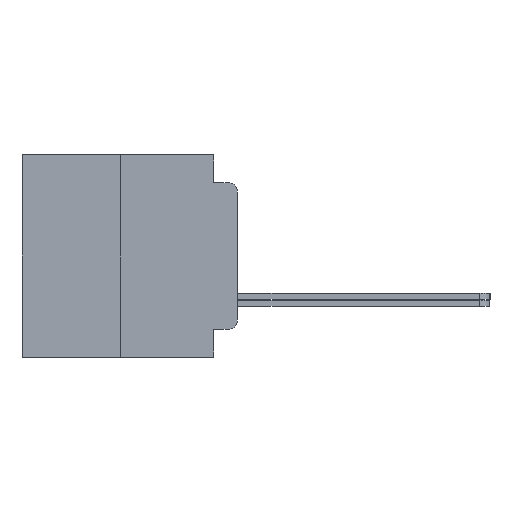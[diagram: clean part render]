
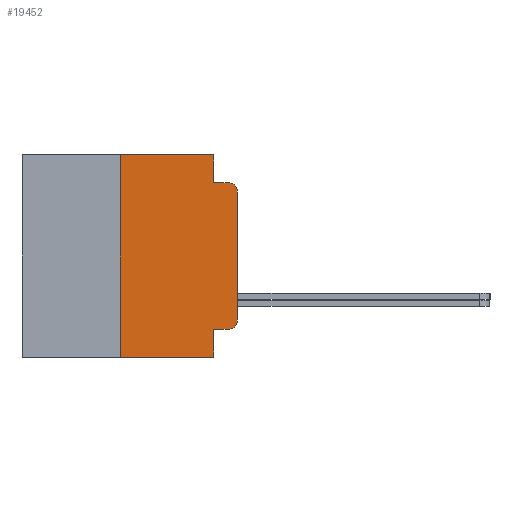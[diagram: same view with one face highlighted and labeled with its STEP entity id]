
A CAD part, left-side view. The second image highlights one B-rep face of the part: STEP entity #19452.
In plain terms, the highlighted planar face has unit normal (-1, 0, 0).
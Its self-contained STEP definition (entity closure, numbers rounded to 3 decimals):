
#220 = VECTOR ( 'NONE', #13989, 1000. ) ;
#304 = VERTEX_POINT ( 'NONE', #727 ) ;
#560 = CARTESIAN_POINT ( 'NONE',  ( -75.603, 0.508, 3.467 ) ) ;
#727 = CARTESIAN_POINT ( 'NONE',  ( -75.603, 1.295, 5.486 ) ) ;
#997 = VERTEX_POINT ( 'NONE', #19934 ) ;
#1401 = CARTESIAN_POINT ( 'NONE',  ( -75.603, 6.35, 5.486 ) ) ;
#2015 = LINE ( 'NONE', #21872, #22476 ) ;
#2050 = LINE ( 'NONE', #23682, #16627 ) ;
#2599 = LINE ( 'NONE', #22266, #8858 ) ;
#2803 = DIRECTION ( 'NONE',  ( 0., 0., -1. ) ) ;
#3021 = LINE ( 'NONE', #4930, #20056 ) ;
#3173 = DIRECTION ( 'NONE',  ( 0., 0., -1. ) ) ;
#4796 = CARTESIAN_POINT ( 'NONE',  ( -75.603, 6.35, -5.486 ) ) ;
#4930 = CARTESIAN_POINT ( 'NONE',  ( -75.603, 0., 5.486 ) ) ;
#5024 = LINE ( 'NONE', #7164, #17158 ) ;
#5097 = VECTOR ( 'NONE', #25494, 1000. ) ;
#5212 = PLANE ( 'NONE',  #24274 ) ;
#5493 = CARTESIAN_POINT ( 'NONE',  ( -75.603, 1.295, -3.975 ) ) ;
#5762 = CARTESIAN_POINT ( 'NONE',  ( -75.603, 1.295, -3.975 ) ) ;
#5811 = EDGE_CURVE ( 'NONE', #6834, #17138, #17463, .T. ) ;
#5921 = CARTESIAN_POINT ( 'NONE',  ( -75.603, 11.684, -5.486 ) ) ;
#6027 = CIRCLE ( 'NONE', #8150, 0.508 ) ;
#6270 = DIRECTION ( 'NONE',  ( 0., 0., -1. ) ) ;
#6372 = DIRECTION ( 'NONE',  ( 0., 0., -1. ) ) ;
#6834 = VERTEX_POINT ( 'NONE', #24407 ) ;
#7164 = CARTESIAN_POINT ( 'NONE',  ( -75.603, 1.295, 3.975 ) ) ;
#7718 = VERTEX_POINT ( 'NONE', #7725 ) ;
#7725 = CARTESIAN_POINT ( 'NONE',  ( -75.603, 0.508, -3.975 ) ) ;
#8150 = AXIS2_PLACEMENT_3D ( 'NONE', #14321, #11889, #3173 ) ;
#8215 = LINE ( 'NONE', #5921, #25603 ) ;
#8858 = VECTOR ( 'NONE', #6372, 1000. ) ;
#9662 = CARTESIAN_POINT ( 'NONE',  ( -75.603, 11.684, 5.486 ) ) ;
#10003 = DIRECTION ( 'NONE',  ( 0., -1., 0. ) ) ;
#10238 = EDGE_CURVE ( 'NONE', #304, #997, #2599, .T. ) ;
#11692 = ORIENTED_EDGE ( 'NONE', *, *, #5811, .T. ) ;
#11889 = DIRECTION ( 'NONE',  ( -1., 0., 0. ) ) ;
#11892 = DIRECTION ( 'NONE',  ( 0., 0., -1. ) ) ;
#12378 = CARTESIAN_POINT ( 'NONE',  ( -75.603, 1.295, -5.486 ) ) ;
#12383 = LINE ( 'NONE', #5493, #5097 ) ;
#12546 = ORIENTED_EDGE ( 'NONE', *, *, #21120, .T. ) ;
#13679 = EDGE_CURVE ( 'NONE', #23875, #15621, #8215, .T. ) ;
#13989 = DIRECTION ( 'NONE',  ( 0., 0., 1. ) ) ;
#14321 = CARTESIAN_POINT ( 'NONE',  ( -75.603, 0.508, -3.467 ) ) ;
#14332 = VERTEX_POINT ( 'NONE', #5762 ) ;
#14363 = VERTEX_POINT ( 'NONE', #1401 ) ;
#14420 = DIRECTION ( 'NONE',  ( 0., -1., 0. ) ) ;
#14686 = EDGE_CURVE ( 'NONE', #997, #17138, #5024, .T. ) ;
#15621 = VERTEX_POINT ( 'NONE', #12378 ) ;
#15919 = ORIENTED_EDGE ( 'NONE', *, *, #14686, .F. ) ;
#16088 = DIRECTION ( 'NONE',  ( -1., 0., 0. ) ) ;
#16627 = VECTOR ( 'NONE', #18845, 1000. ) ;
#17138 = VERTEX_POINT ( 'NONE', #26164 ) ;
#17158 = VECTOR ( 'NONE', #14420, 1000. ) ;
#17463 = CIRCLE ( 'NONE', #21462, 0.508 ) ;
#17610 = EDGE_CURVE ( 'NONE', #14363, #304, #2050, .T. ) ;
#18006 = ORIENTED_EDGE ( 'NONE', *, *, #21700, .F. ) ;
#18749 = VERTEX_POINT ( 'NONE', #21094 ) ;
#18845 = DIRECTION ( 'NONE',  ( 0., -1., 0. ) ) ;
#18940 = EDGE_CURVE ( 'NONE', #14332, #15621, #2015, .T. ) ;
#19056 = ORIENTED_EDGE ( 'NONE', *, *, #10238, .F. ) ;
#19164 = ORIENTED_EDGE ( 'NONE', *, *, #21260, .T. ) ;
#19452 = ADVANCED_FACE ( 'NONE', ( #22907 ), #5212, .F. ) ;
#19681 = ORIENTED_EDGE ( 'NONE', *, *, #23400, .T. ) ;
#19934 = CARTESIAN_POINT ( 'NONE',  ( -75.603, 1.295, 3.975 ) ) ;
#20056 = VECTOR ( 'NONE', #22746, 1000. ) ;
#21094 = CARTESIAN_POINT ( 'NONE',  ( -75.603, 0., -3.467 ) ) ;
#21120 = EDGE_CURVE ( 'NONE', #18749, #6834, #3021, .T. ) ;
#21260 = EDGE_CURVE ( 'NONE', #14332, #7718, #12383, .T. ) ;
#21462 = AXIS2_PLACEMENT_3D ( 'NONE', #560, #16088, #2803 ) ;
#21700 = EDGE_CURVE ( 'NONE', #23875, #14363, #26977, .T. ) ;
#21872 = CARTESIAN_POINT ( 'NONE',  ( -75.603, 1.295, 0. ) ) ;
#22266 = CARTESIAN_POINT ( 'NONE',  ( -75.603, 1.295, 0. ) ) ;
#22476 = VECTOR ( 'NONE', #6270, 1000. ) ;
#22710 = CARTESIAN_POINT ( 'NONE',  ( -75.603, 6.35, -5.486 ) ) ;
#22746 = DIRECTION ( 'NONE',  ( 0., 0., 1. ) ) ;
#22907 = FACE_OUTER_BOUND ( 'NONE', #25120, .T. ) ;
#23400 = EDGE_CURVE ( 'NONE', #7718, #18749, #6027, .T. ) ;
#23682 = CARTESIAN_POINT ( 'NONE',  ( -75.603, 11.684, 5.486 ) ) ;
#23875 = VERTEX_POINT ( 'NONE', #4796 ) ;
#23933 = ORIENTED_EDGE ( 'NONE', *, *, #17610, .F. ) ;
#24274 = AXIS2_PLACEMENT_3D ( 'NONE', #9662, #25194, #11892 ) ;
#24407 = CARTESIAN_POINT ( 'NONE',  ( -75.603, 0., 3.467 ) ) ;
#25120 = EDGE_LOOP ( 'NONE', ( #19164, #19681, #12546, #11692, #15919, #19056, #23933, #18006, #28567, #28282 ) ) ;
#25194 = DIRECTION ( 'NONE',  ( 1., 0., 0. ) ) ;
#25494 = DIRECTION ( 'NONE',  ( 0., -1., 0. ) ) ;
#25603 = VECTOR ( 'NONE', #10003, 1000. ) ;
#26164 = CARTESIAN_POINT ( 'NONE',  ( -75.603, 0.508, 3.975 ) ) ;
#26977 = LINE ( 'NONE', #22710, #220 ) ;
#28282 = ORIENTED_EDGE ( 'NONE', *, *, #18940, .F. ) ;
#28567 = ORIENTED_EDGE ( 'NONE', *, *, #13679, .T. ) ;
